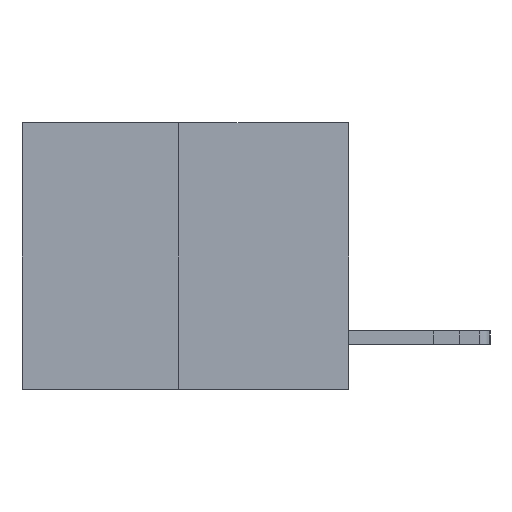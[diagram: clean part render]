
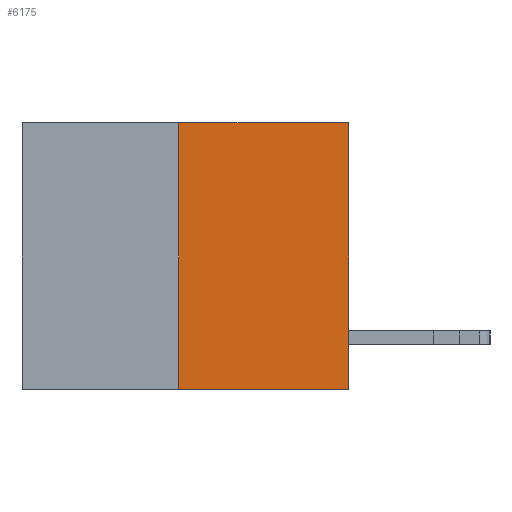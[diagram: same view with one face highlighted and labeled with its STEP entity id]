
A CAD part, left-side view. The second image highlights one B-rep face of the part: STEP entity #6175.
In plain terms, the highlighted planar face has unit normal (-1, 0, 0).
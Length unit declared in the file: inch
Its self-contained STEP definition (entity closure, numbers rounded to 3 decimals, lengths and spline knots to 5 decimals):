
#106 = PLANE ( 'NONE',  #8781 ) ;
#271 = DIRECTION ( 'NONE',  ( 0., 0., -1. ) ) ;
#662 = VERTEX_POINT ( 'NONE', #15649 ) ;
#1130 = LINE ( 'NONE', #8609, #10460 ) ;
#1161 = DIRECTION ( 'NONE',  ( 0., 0., 1. ) ) ;
#1232 = VERTEX_POINT ( 'NONE', #8743 ) ;
#1484 = DIRECTION ( 'NONE',  ( 1., 0., 0. ) ) ;
#1670 = EDGE_CURVE ( 'NONE', #1232, #9409, #1130, .T. ) ;
#1927 = EDGE_CURVE ( 'NONE', #5130, #9409, #14795, .T. ) ;
#2067 = VECTOR ( 'NONE', #13968, 39.37008 ) ;
#2815 = ORIENTED_EDGE ( 'NONE', *, *, #1670, .T. ) ;
#3395 = EDGE_LOOP ( 'NONE', ( #10342, #12745, #2815, #11843 ) ) ;
#3751 = CARTESIAN_POINT ( 'NONE',  ( 0., 0.312, 0. ) ) ;
#3767 = CARTESIAN_POINT ( 'NONE',  ( 0., 0., 0. ) ) ;
#5130 = VERTEX_POINT ( 'NONE', #3751 ) ;
#5885 = EDGE_CURVE ( 'NONE', #662, #1232, #15281, .T. ) ;
#6175 = ADVANCED_FACE ( 'NONE', ( #10547 ), #106, .F. ) ;
#6728 = CARTESIAN_POINT ( 'NONE',  ( 0., 0.6, -0.49 ) ) ;
#6791 = CARTESIAN_POINT ( 'NONE',  ( 0., 0.6, 0. ) ) ;
#6997 = DIRECTION ( 'NONE',  ( 0., -1., 0. ) ) ;
#7737 = CARTESIAN_POINT ( 'NONE',  ( 0., 0.6, 0. ) ) ;
#8609 = CARTESIAN_POINT ( 'NONE',  ( 0., 0., 0. ) ) ;
#8618 = VECTOR ( 'NONE', #9287, 39.37008 ) ;
#8743 = CARTESIAN_POINT ( 'NONE',  ( 0., 0., -0.49 ) ) ;
#8781 = AXIS2_PLACEMENT_3D ( 'NONE', #7737, #1484, #271 ) ;
#9024 = CARTESIAN_POINT ( 'NONE',  ( 0., 0.312, -0.49 ) ) ;
#9287 = DIRECTION ( 'NONE',  ( 0., -1., 0. ) ) ;
#9409 = VERTEX_POINT ( 'NONE', #3767 ) ;
#10342 = ORIENTED_EDGE ( 'NONE', *, *, #11667, .F. ) ;
#10460 = VECTOR ( 'NONE', #1161, 39.37008 ) ;
#10547 = FACE_OUTER_BOUND ( 'NONE', #3395, .T. ) ;
#11667 = EDGE_CURVE ( 'NONE', #662, #5130, #15358, .T. ) ;
#11843 = ORIENTED_EDGE ( 'NONE', *, *, #1927, .F. ) ;
#12016 = VECTOR ( 'NONE', #6997, 39.37008 ) ;
#12745 = ORIENTED_EDGE ( 'NONE', *, *, #5885, .T. ) ;
#13968 = DIRECTION ( 'NONE',  ( 0., 0., 1. ) ) ;
#14795 = LINE ( 'NONE', #6791, #12016 ) ;
#15281 = LINE ( 'NONE', #6728, #8618 ) ;
#15358 = LINE ( 'NONE', #9024, #2067 ) ;
#15649 = CARTESIAN_POINT ( 'NONE',  ( 0., 0.312, -0.49 ) ) ;
